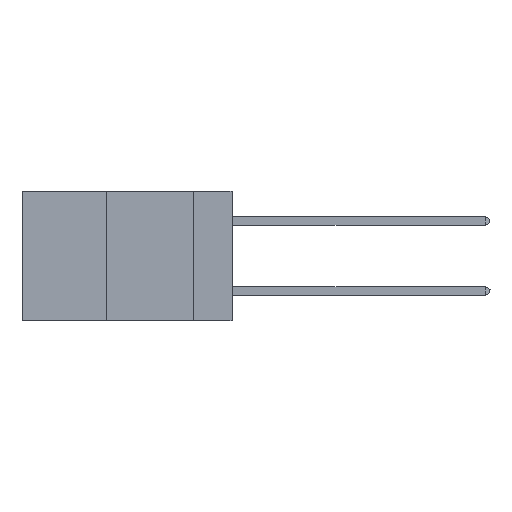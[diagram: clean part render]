
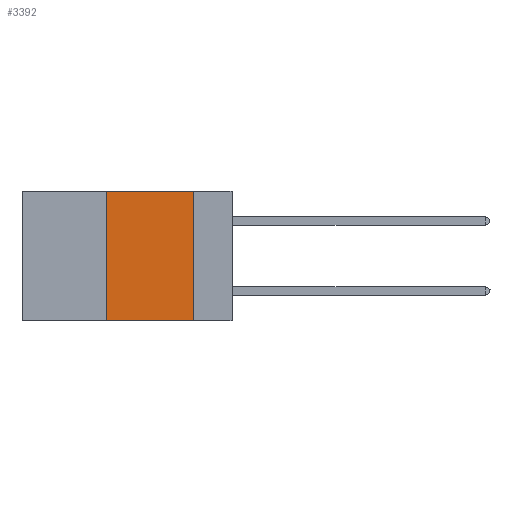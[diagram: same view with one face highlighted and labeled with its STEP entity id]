
A CAD part, left-side view. The second image highlights one B-rep face of the part: STEP entity #3392.
In plain terms, the highlighted planar face has unit normal (-1, 0, 0).
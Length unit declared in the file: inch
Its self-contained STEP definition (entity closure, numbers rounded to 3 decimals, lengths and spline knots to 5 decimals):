
#337 = CARTESIAN_POINT ( 'NONE',  ( 0., 0.11, 0. ) ) ;
#1585 = DIRECTION ( 'NONE',  ( 0., 0., -1. ) ) ;
#1824 = CARTESIAN_POINT ( 'NONE',  ( 0., 0.6, 0. ) ) ;
#2498 = CARTESIAN_POINT ( 'NONE',  ( 0., 0.6, -0.37 ) ) ;
#2968 = EDGE_CURVE ( 'NONE', #5156, #14504, #15495, .T. ) ;
#3392 = ADVANCED_FACE ( 'NONE', ( #16514 ), #8933, .F. ) ;
#3437 = EDGE_CURVE ( 'NONE', #5156, #15381, #9009, .T. ) ;
#4466 = DIRECTION ( 'NONE',  ( 0., -1., 0. ) ) ;
#5074 = DIRECTION ( 'NONE',  ( 0., 0., -1. ) ) ;
#5156 = VERTEX_POINT ( 'NONE', #17203 ) ;
#5473 = EDGE_CURVE ( 'NONE', #10525, #15381, #6359, .T. ) ;
#6071 = VECTOR ( 'NONE', #7909, 39.37008 ) ;
#6359 = LINE ( 'NONE', #337, #7392 ) ;
#7160 = ORIENTED_EDGE ( 'NONE', *, *, #5473, .F. ) ;
#7284 = DIRECTION ( 'NONE',  ( 1., 0., 0. ) ) ;
#7296 = ORIENTED_EDGE ( 'NONE', *, *, #2968, .F. ) ;
#7345 = EDGE_CURVE ( 'NONE', #14504, #10525, #15078, .T. ) ;
#7392 = VECTOR ( 'NONE', #1585, 39.37008 ) ;
#7909 = DIRECTION ( 'NONE',  ( 0., 0., 1. ) ) ;
#8807 = CARTESIAN_POINT ( 'NONE',  ( 0., 0.36, 0. ) ) ;
#8845 = AXIS2_PLACEMENT_3D ( 'NONE', #1824, #7284, #5074 ) ;
#8933 = PLANE ( 'NONE',  #8845 ) ;
#9009 = LINE ( 'NONE', #2498, #12740 ) ;
#9050 = CARTESIAN_POINT ( 'NONE',  ( 0., 0.36, 0. ) ) ;
#9718 = DIRECTION ( 'NONE',  ( 0., -1., 0. ) ) ;
#10362 = ORIENTED_EDGE ( 'NONE', *, *, #7345, .F. ) ;
#10525 = VERTEX_POINT ( 'NONE', #13999 ) ;
#10714 = CARTESIAN_POINT ( 'NONE',  ( 0., 0.6, 0. ) ) ;
#12140 = VECTOR ( 'NONE', #9718, 39.37008 ) ;
#12175 = ORIENTED_EDGE ( 'NONE', *, *, #3437, .T. ) ;
#12740 = VECTOR ( 'NONE', #4466, 39.37008 ) ;
#13673 = CARTESIAN_POINT ( 'NONE',  ( 0., 0.11, -0.37 ) ) ;
#13999 = CARTESIAN_POINT ( 'NONE',  ( 0., 0.11, 0. ) ) ;
#14504 = VERTEX_POINT ( 'NONE', #8807 ) ;
#15078 = LINE ( 'NONE', #10714, #12140 ) ;
#15381 = VERTEX_POINT ( 'NONE', #13673 ) ;
#15495 = LINE ( 'NONE', #9050, #6071 ) ;
#16514 = FACE_OUTER_BOUND ( 'NONE', #16810, .T. ) ;
#16810 = EDGE_LOOP ( 'NONE', ( #7160, #10362, #7296, #12175 ) ) ;
#17203 = CARTESIAN_POINT ( 'NONE',  ( 0., 0.36, -0.37 ) ) ;
